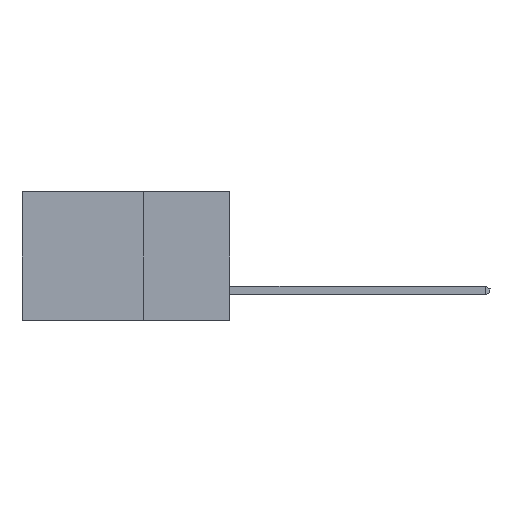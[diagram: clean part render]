
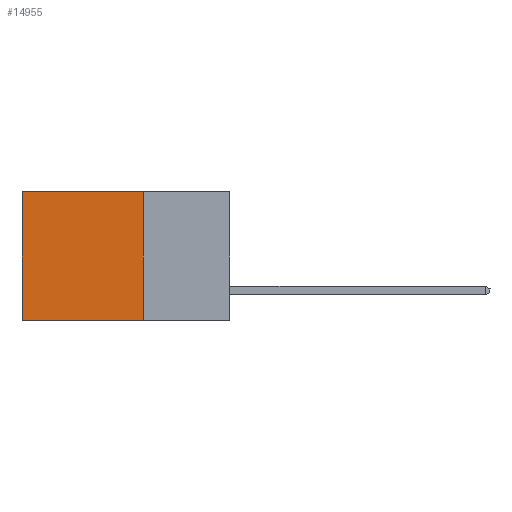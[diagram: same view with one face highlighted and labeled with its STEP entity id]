
A CAD part, left-side view. The second image highlights one B-rep face of the part: STEP entity #14955.
In plain terms, the highlighted planar face has unit normal (-1, 0, 0).
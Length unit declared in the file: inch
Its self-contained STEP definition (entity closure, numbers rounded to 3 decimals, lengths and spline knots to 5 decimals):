
#958 = VECTOR ( 'NONE', #19145, 39.37008 ) ;
#1433 = VERTEX_POINT ( 'NONE', #10155 ) ;
#1627 = EDGE_CURVE ( 'NONE', #1433, #12255, #20135, .T. ) ;
#1696 = EDGE_CURVE ( 'NONE', #6844, #1433, #19356, .T. ) ;
#2110 = CARTESIAN_POINT ( 'NONE',  ( 0.2615, 0.25, -0.37 ) ) ;
#2639 = DIRECTION ( 'NONE',  ( 0., 1., 0. ) ) ;
#3021 = VECTOR ( 'NONE', #3300, 39.37008 ) ;
#3300 = DIRECTION ( 'NONE',  ( 0., 1., 0. ) ) ;
#4619 = EDGE_CURVE ( 'NONE', #6844, #16852, #17298, .T. ) ;
#5619 = DIRECTION ( 'NONE',  ( 1., 0., 0. ) ) ;
#6007 = EDGE_CURVE ( 'NONE', #16852, #12255, #19132, .T. ) ;
#6231 = CARTESIAN_POINT ( 'NONE',  ( 0.2615, 0.25, 0. ) ) ;
#6844 = VERTEX_POINT ( 'NONE', #14718 ) ;
#7249 = FACE_OUTER_BOUND ( 'NONE', #10289, .T. ) ;
#7442 = DIRECTION ( 'NONE',  ( 0., 0., -1. ) ) ;
#7619 = VECTOR ( 'NONE', #7442, 39.37008 ) ;
#8674 = ORIENTED_EDGE ( 'NONE', *, *, #4619, .F. ) ;
#9183 = CARTESIAN_POINT ( 'NONE',  ( 0.2615, 0.25, -0.37 ) ) ;
#10137 = CARTESIAN_POINT ( 'NONE',  ( 0.2615, 0.6, -0.37 ) ) ;
#10155 = CARTESIAN_POINT ( 'NONE',  ( 0.2615, 0.6, 0. ) ) ;
#10289 = EDGE_LOOP ( 'NONE', ( #11133, #14247, #8674, #19681 ) ) ;
#10769 = VECTOR ( 'NONE', #2639, 39.37008 ) ;
#10890 = CARTESIAN_POINT ( 'NONE',  ( 0.2615, 0.25, -0.37 ) ) ;
#11133 = ORIENTED_EDGE ( 'NONE', *, *, #1627, .T. ) ;
#12255 = VERTEX_POINT ( 'NONE', #10137 ) ;
#12336 = DIRECTION ( 'NONE',  ( 0., 0., -1. ) ) ;
#12525 = CARTESIAN_POINT ( 'NONE',  ( 0.2615, 0.6, -0.37 ) ) ;
#14247 = ORIENTED_EDGE ( 'NONE', *, *, #6007, .F. ) ;
#14718 = CARTESIAN_POINT ( 'NONE',  ( 0.2615, 0.25, 0. ) ) ;
#14955 = ADVANCED_FACE ( 'NONE', ( #7249 ), #18624, .F. ) ;
#16852 = VERTEX_POINT ( 'NONE', #9183 ) ;
#17298 = LINE ( 'NONE', #2110, #7619 ) ;
#18624 = PLANE ( 'NONE',  #18988 ) ;
#18988 = AXIS2_PLACEMENT_3D ( 'NONE', #20261, #5619, #12336 ) ;
#19132 = LINE ( 'NONE', #10890, #10769 ) ;
#19145 = DIRECTION ( 'NONE',  ( 0., 0., -1. ) ) ;
#19356 = LINE ( 'NONE', #6231, #3021 ) ;
#19681 = ORIENTED_EDGE ( 'NONE', *, *, #1696, .T. ) ;
#20135 = LINE ( 'NONE', #12525, #958 ) ;
#20261 = CARTESIAN_POINT ( 'NONE',  ( 0.2615, 0.25, -0.37 ) ) ;
